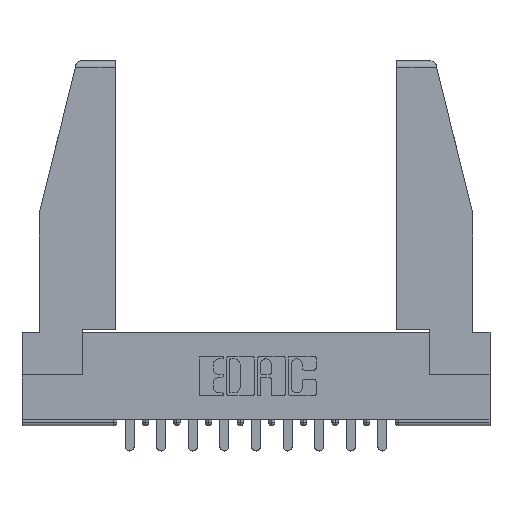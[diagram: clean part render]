
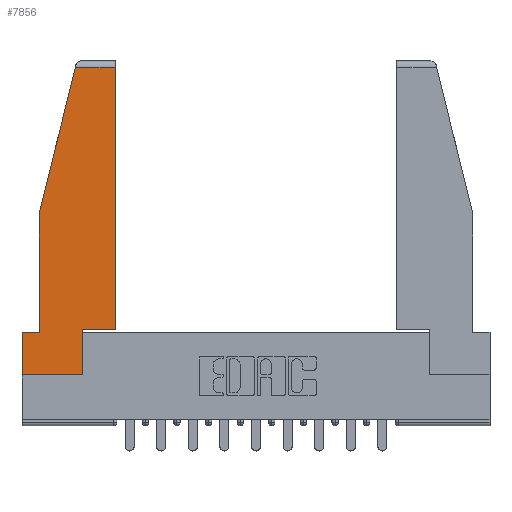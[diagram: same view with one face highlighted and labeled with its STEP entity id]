
A CAD part, top view. The second image highlights one B-rep face of the part: STEP entity #7856.
In plain terms, the highlighted planar face has unit normal (0, 0, 1).
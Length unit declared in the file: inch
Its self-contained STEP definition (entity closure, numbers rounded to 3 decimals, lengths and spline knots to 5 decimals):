
#586 = DIRECTION ( 'NONE',  ( -0.239, -0.971, 0. ) ) ;
#887 = CARTESIAN_POINT ( 'NONE',  ( 0.086, 0.8, 0. ) ) ;
#1525 = DIRECTION ( 'NONE',  ( 0., -1., 0. ) ) ;
#1592 = CARTESIAN_POINT ( 'NONE',  ( 0.297, 0.223, 0. ) ) ;
#1958 = EDGE_CURVE ( 'NONE', #4590, #2628, #11077, .T. ) ;
#2073 = ORIENTED_EDGE ( 'NONE', *, *, #9964, .T. ) ;
#2224 = ORIENTED_EDGE ( 'NONE', *, *, #1958, .T. ) ;
#2628 = VERTEX_POINT ( 'NONE', #11691 ) ;
#2657 = LINE ( 'NONE', #15176, #10277 ) ;
#2878 = ORIENTED_EDGE ( 'NONE', *, *, #3681, .T. ) ;
#2939 = AXIS2_PLACEMENT_3D ( 'NONE', #15466, #8053, #11736 ) ;
#2946 = EDGE_CURVE ( 'NONE', #6206, #4590, #6960, .T. ) ;
#3360 = EDGE_CURVE ( 'NONE', #15535, #8891, #4383, .T. ) ;
#3456 = CARTESIAN_POINT ( 'NONE',  ( 0., 0., 0. ) ) ;
#3681 = EDGE_CURVE ( 'NONE', #6675, #5174, #15260, .T. ) ;
#3905 = FACE_OUTER_BOUND ( 'NONE', #15677, .T. ) ;
#4001 = PLANE ( 'NONE',  #2939 ) ;
#4383 = LINE ( 'NONE', #14636, #13351 ) ;
#4456 = EDGE_CURVE ( 'NONE', #8891, #5640, #9236, .T. ) ;
#4590 = VERTEX_POINT ( 'NONE', #13070 ) ;
#4873 = ORIENTED_EDGE ( 'NONE', *, *, #11390, .T. ) ;
#5174 = VERTEX_POINT ( 'NONE', #9489 ) ;
#5240 = VECTOR ( 'NONE', #15551, 39.37008 ) ;
#5624 = CARTESIAN_POINT ( 'NONE',  ( 0.461, 0.223, 0. ) ) ;
#5640 = VERTEX_POINT ( 'NONE', #6706 ) ;
#5915 = CARTESIAN_POINT ( 'NONE',  ( 0.297, 0., 0. ) ) ;
#6132 = CARTESIAN_POINT ( 'NONE',  ( 0., 1.52, 0. ) ) ;
#6206 = VERTEX_POINT ( 'NONE', #7121 ) ;
#6553 = ORIENTED_EDGE ( 'NONE', *, *, #11296, .T. ) ;
#6560 = LINE ( 'NONE', #5915, #15273 ) ;
#6675 = VERTEX_POINT ( 'NONE', #11958 ) ;
#6706 = CARTESIAN_POINT ( 'NONE',  ( 0., 0.21, 0. ) ) ;
#6960 = LINE ( 'NONE', #1592, #12028 ) ;
#7121 = CARTESIAN_POINT ( 'NONE',  ( 0.297, 0.223, 0. ) ) ;
#7592 = CARTESIAN_POINT ( 'NONE',  ( 0.086, 0.21, 0. ) ) ;
#7856 = ADVANCED_FACE ( 'NONE', ( #3905 ), #4001, .T. ) ;
#7905 = CARTESIAN_POINT ( 'NONE',  ( 0.271, 1.55, 0. ) ) ;
#7962 = ORIENTED_EDGE ( 'NONE', *, *, #3360, .T. ) ;
#8053 = DIRECTION ( 'NONE',  ( 0., 0., 1. ) ) ;
#8096 = ORIENTED_EDGE ( 'NONE', *, *, #10473, .T. ) ;
#8299 = VECTOR ( 'NONE', #9764, 39.37008 ) ;
#8712 = VECTOR ( 'NONE', #14768, 39.37008 ) ;
#8718 = ORIENTED_EDGE ( 'NONE', *, *, #2946, .T. ) ;
#8891 = VERTEX_POINT ( 'NONE', #7592 ) ;
#8921 = DIRECTION ( 'NONE',  ( 1., 0., 0. ) ) ;
#9040 = VECTOR ( 'NONE', #14096, 39.37008 ) ;
#9236 = LINE ( 'NONE', #10421, #9040 ) ;
#9489 = CARTESIAN_POINT ( 'NONE',  ( 0.297, 0., 0. ) ) ;
#9764 = DIRECTION ( 'NONE',  ( 1., 0., 0. ) ) ;
#9816 = DIRECTION ( 'NONE',  ( 0., -1., 0. ) ) ;
#9960 = ORIENTED_EDGE ( 'NONE', *, *, #4456, .T. ) ;
#9964 = EDGE_CURVE ( 'NONE', #13465, #15535, #15733, .T. ) ;
#10277 = VECTOR ( 'NONE', #1525, 39.37008 ) ;
#10421 = CARTESIAN_POINT ( 'NONE',  ( 0., 0.21, 0. ) ) ;
#10473 = EDGE_CURVE ( 'NONE', #5640, #6675, #2657, .T. ) ;
#11077 = LINE ( 'NONE', #5624, #5240 ) ;
#11296 = EDGE_CURVE ( 'NONE', #5174, #6206, #6560, .T. ) ;
#11390 = EDGE_CURVE ( 'NONE', #2628, #13465, #16067, .T. ) ;
#11691 = CARTESIAN_POINT ( 'NONE',  ( 0.461, 1.52, 0. ) ) ;
#11736 = DIRECTION ( 'NONE',  ( 1., 0., 0. ) ) ;
#11958 = CARTESIAN_POINT ( 'NONE',  ( 0., 0., 0. ) ) ;
#12028 = VECTOR ( 'NONE', #8921, 39.37008 ) ;
#12078 = VECTOR ( 'NONE', #586, 39.37008 ) ;
#13070 = CARTESIAN_POINT ( 'NONE',  ( 0.461, 0.223, 0. ) ) ;
#13351 = VECTOR ( 'NONE', #9816, 39.37008 ) ;
#13465 = VERTEX_POINT ( 'NONE', #13921 ) ;
#13921 = CARTESIAN_POINT ( 'NONE',  ( 0.2636, 1.52, 0. ) ) ;
#14096 = DIRECTION ( 'NONE',  ( -1., 0., 0. ) ) ;
#14636 = CARTESIAN_POINT ( 'NONE',  ( 0.086, 0.8, 0. ) ) ;
#14768 = DIRECTION ( 'NONE',  ( -1., 0., 0. ) ) ;
#15176 = CARTESIAN_POINT ( 'NONE',  ( 0., 0.21, 0. ) ) ;
#15260 = LINE ( 'NONE', #3456, #8299 ) ;
#15273 = VECTOR ( 'NONE', #15847, 39.37008 ) ;
#15466 = CARTESIAN_POINT ( 'NONE',  ( 0., 0., 0. ) ) ;
#15535 = VERTEX_POINT ( 'NONE', #887 ) ;
#15551 = DIRECTION ( 'NONE',  ( 0., 1., 0. ) ) ;
#15677 = EDGE_LOOP ( 'NONE', ( #2224, #4873, #2073, #7962, #9960, #8096, #2878, #6553, #8718 ) ) ;
#15733 = LINE ( 'NONE', #7905, #12078 ) ;
#15847 = DIRECTION ( 'NONE',  ( 0., 1., 0. ) ) ;
#16067 = LINE ( 'NONE', #6132, #8712 ) ;
